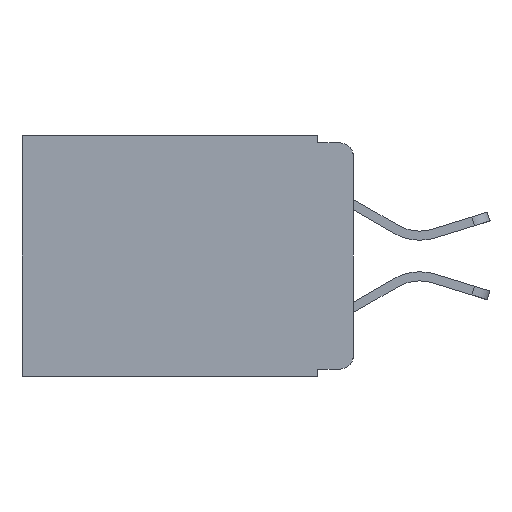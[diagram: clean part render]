
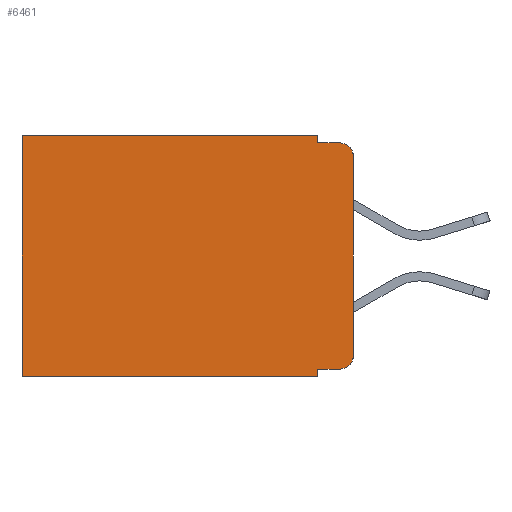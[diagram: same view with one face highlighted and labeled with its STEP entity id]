
A CAD part, left-side view. The second image highlights one B-rep face of the part: STEP entity #6461.
In plain terms, the highlighted planar face has unit normal (-1, 0, 0).
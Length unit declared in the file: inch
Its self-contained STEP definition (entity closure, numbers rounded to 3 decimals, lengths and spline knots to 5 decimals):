
#200 = DIRECTION ( 'NONE',  ( 0., -1., 0. ) ) ;
#320 = CARTESIAN_POINT ( 'NONE',  ( 0.298, 0.051, 0. ) ) ;
#339 = LINE ( 'NONE', #6530, #11680 ) ;
#882 = DIRECTION ( 'NONE',  ( 0., 0., -1. ) ) ;
#1149 = EDGE_CURVE ( 'NONE', #8418, #6369, #6676, .T. ) ;
#1171 = VERTEX_POINT ( 'NONE', #8475 ) ;
#1292 = CARTESIAN_POINT ( 'NONE',  ( 0.298, 0.051, 0. ) ) ;
#1312 = EDGE_CURVE ( 'NONE', #5210, #13140, #20109, .T. ) ;
#1605 = VECTOR ( 'NONE', #4675, 39.37008 ) ;
#1645 = VECTOR ( 'NONE', #19662, 39.37008 ) ;
#1864 = CARTESIAN_POINT ( 'NONE',  ( 0.298, 0.051, -0.333 ) ) ;
#1946 = EDGE_LOOP ( 'NONE', ( #7581, #2339, #6474, #12672, #19264, #15922, #11283, #5335, #8498, #18564 ) ) ;
#2339 = ORIENTED_EDGE ( 'NONE', *, *, #4014, .T. ) ;
#2676 = CARTESIAN_POINT ( 'NONE',  ( 0.298, 0.051, -0.01 ) ) ;
#3119 = CARTESIAN_POINT ( 'NONE',  ( 0.298, 0.473, -0.343 ) ) ;
#3199 = PLANE ( 'NONE',  #7218 ) ;
#3565 = AXIS2_PLACEMENT_3D ( 'NONE', #7714, #18482, #9282 ) ;
#4014 = EDGE_CURVE ( 'NONE', #19540, #12190, #8789, .T. ) ;
#4289 = EDGE_CURVE ( 'NONE', #6239, #5210, #12228, .T. ) ;
#4434 = DIRECTION ( 'NONE',  ( 0., 1., 0. ) ) ;
#4651 = VERTEX_POINT ( 'NONE', #2676 ) ;
#4675 = DIRECTION ( 'NONE',  ( 0., 0., -1. ) ) ;
#4854 = CARTESIAN_POINT ( 'NONE',  ( 0.298, 0., 0. ) ) ;
#5186 = VECTOR ( 'NONE', #11213, 39.37008 ) ;
#5210 = VERTEX_POINT ( 'NONE', #13552 ) ;
#5307 = CARTESIAN_POINT ( 'NONE',  ( 0.298, 0., -0.313 ) ) ;
#5335 = ORIENTED_EDGE ( 'NONE', *, *, #7605, .F. ) ;
#5960 = EDGE_CURVE ( 'NONE', #8418, #4651, #10671, .T. ) ;
#6030 = CARTESIAN_POINT ( 'NONE',  ( 0.298, 0., 0. ) ) ;
#6239 = VERTEX_POINT ( 'NONE', #15191 ) ;
#6369 = VERTEX_POINT ( 'NONE', #9323 ) ;
#6375 = VECTOR ( 'NONE', #12258, 39.37008 ) ;
#6461 = ADVANCED_FACE ( 'NONE', ( #17356 ), #3199, .F. ) ;
#6465 = VERTEX_POINT ( 'NONE', #3119 ) ;
#6469 = DIRECTION ( 'NONE',  ( 0., 0., -1. ) ) ;
#6474 = ORIENTED_EDGE ( 'NONE', *, *, #11061, .F. ) ;
#6530 = CARTESIAN_POINT ( 'NONE',  ( 0.298, 0.051, -0.01 ) ) ;
#6570 = EDGE_CURVE ( 'NONE', #1171, #6465, #8180, .T. ) ;
#6676 = LINE ( 'NONE', #6937, #18966 ) ;
#6937 = CARTESIAN_POINT ( 'NONE',  ( 0.298, 0., 0. ) ) ;
#7099 = CARTESIAN_POINT ( 'NONE',  ( 0.298, 0., -0.03 ) ) ;
#7218 = AXIS2_PLACEMENT_3D ( 'NONE', #4854, #15758, #6469 ) ;
#7581 = ORIENTED_EDGE ( 'NONE', *, *, #15110, .F. ) ;
#7605 = EDGE_CURVE ( 'NONE', #6239, #1171, #13520, .T. ) ;
#7714 = CARTESIAN_POINT ( 'NONE',  ( 0.298, 0.02, -0.03 ) ) ;
#8079 = DIRECTION ( 'NONE',  ( 0., -1., 0. ) ) ;
#8180 = LINE ( 'NONE', #19048, #19925 ) ;
#8418 = VERTEX_POINT ( 'NONE', #320 ) ;
#8463 = DIRECTION ( 'NONE',  ( -1., 0., 0. ) ) ;
#8475 = CARTESIAN_POINT ( 'NONE',  ( 0.298, 0.051, -0.343 ) ) ;
#8498 = ORIENTED_EDGE ( 'NONE', *, *, #4289, .T. ) ;
#8789 = CIRCLE ( 'NONE', #3565, 0.02 ) ;
#9282 = DIRECTION ( 'NONE',  ( 0., 0., -1. ) ) ;
#9323 = CARTESIAN_POINT ( 'NONE',  ( 0.298, 0.473, 0. ) ) ;
#9619 = CARTESIAN_POINT ( 'NONE',  ( 0.298, 0.051, 0. ) ) ;
#9713 = LINE ( 'NONE', #10541, #1645 ) ;
#10541 = CARTESIAN_POINT ( 'NONE',  ( 0.298, 0.473, 0. ) ) ;
#10639 = CARTESIAN_POINT ( 'NONE',  ( 0.298, 0.02, -0.313 ) ) ;
#10671 = LINE ( 'NONE', #1292, #1605 ) ;
#11061 = EDGE_CURVE ( 'NONE', #4651, #12190, #339, .T. ) ;
#11213 = DIRECTION ( 'NONE',  ( 0., 0., -1. ) ) ;
#11283 = ORIENTED_EDGE ( 'NONE', *, *, #6570, .F. ) ;
#11366 = AXIS2_PLACEMENT_3D ( 'NONE', #10639, #8463, #882 ) ;
#11419 = EDGE_CURVE ( 'NONE', #6369, #6465, #9713, .T. ) ;
#11680 = VECTOR ( 'NONE', #8079, 39.37008 ) ;
#12190 = VERTEX_POINT ( 'NONE', #15247 ) ;
#12228 = LINE ( 'NONE', #1864, #15805 ) ;
#12258 = DIRECTION ( 'NONE',  ( 0., 0., -1. ) ) ;
#12672 = ORIENTED_EDGE ( 'NONE', *, *, #5960, .F. ) ;
#13140 = VERTEX_POINT ( 'NONE', #5307 ) ;
#13520 = LINE ( 'NONE', #9619, #5186 ) ;
#13552 = CARTESIAN_POINT ( 'NONE',  ( 0.298, 0.02, -0.333 ) ) ;
#14673 = LINE ( 'NONE', #6030, #6375 ) ;
#15110 = EDGE_CURVE ( 'NONE', #19540, #13140, #14673, .T. ) ;
#15191 = CARTESIAN_POINT ( 'NONE',  ( 0.298, 0.051, -0.333 ) ) ;
#15247 = CARTESIAN_POINT ( 'NONE',  ( 0.298, 0.02, -0.01 ) ) ;
#15758 = DIRECTION ( 'NONE',  ( 1., 0., 0. ) ) ;
#15805 = VECTOR ( 'NONE', #200, 39.37008 ) ;
#15922 = ORIENTED_EDGE ( 'NONE', *, *, #11419, .T. ) ;
#16000 = DIRECTION ( 'NONE',  ( 0., 1., 0. ) ) ;
#17356 = FACE_OUTER_BOUND ( 'NONE', #1946, .T. ) ;
#18482 = DIRECTION ( 'NONE',  ( -1., 0., 0. ) ) ;
#18564 = ORIENTED_EDGE ( 'NONE', *, *, #1312, .T. ) ;
#18966 = VECTOR ( 'NONE', #4434, 39.37008 ) ;
#19048 = CARTESIAN_POINT ( 'NONE',  ( 0.298, 0., -0.343 ) ) ;
#19264 = ORIENTED_EDGE ( 'NONE', *, *, #1149, .T. ) ;
#19540 = VERTEX_POINT ( 'NONE', #7099 ) ;
#19662 = DIRECTION ( 'NONE',  ( 0., 0., -1. ) ) ;
#19925 = VECTOR ( 'NONE', #16000, 39.37008 ) ;
#20109 = CIRCLE ( 'NONE', #11366, 0.02 ) ;
